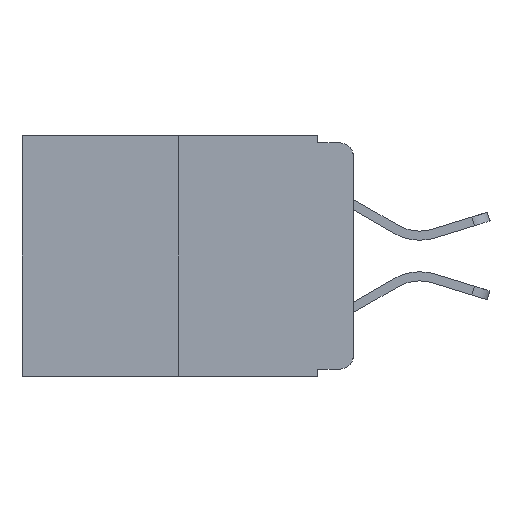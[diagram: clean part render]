
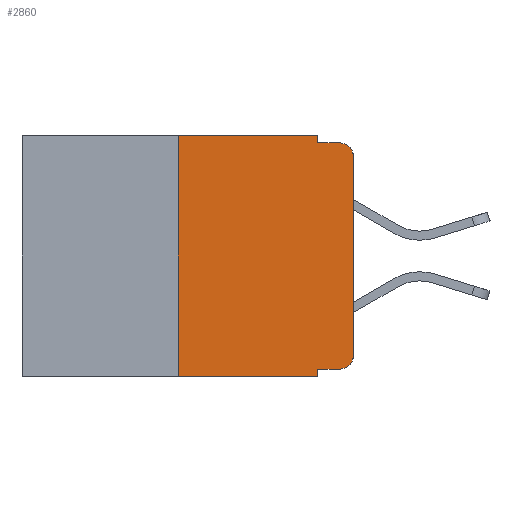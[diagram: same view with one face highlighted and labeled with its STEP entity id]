
A CAD part, left-side view. The second image highlights one B-rep face of the part: STEP entity #2860.
In plain terms, the highlighted planar face has unit normal (-1, 0, 0).
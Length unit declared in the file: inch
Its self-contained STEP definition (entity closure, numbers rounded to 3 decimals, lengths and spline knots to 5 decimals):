
#567 = EDGE_CURVE ( 'NONE', #4420, #1802, #23618, .T. ) ;
#629 = DIRECTION ( 'NONE',  ( 0., -1., 0. ) ) ;
#765 = VECTOR ( 'NONE', #10730, 39.37008 ) ;
#937 = DIRECTION ( 'NONE',  ( 0., -1., 0. ) ) ;
#1701 = DIRECTION ( 'NONE',  ( 0., 0., -1. ) ) ;
#1780 = PLANE ( 'NONE',  #20374 ) ;
#1802 = VERTEX_POINT ( 'NONE', #21354 ) ;
#2081 = VERTEX_POINT ( 'NONE', #8287 ) ;
#2464 = CARTESIAN_POINT ( 'NONE',  ( 0., 0.25, 0. ) ) ;
#2860 = ADVANCED_FACE ( 'NONE', ( #14733 ), #1780, .F. ) ;
#2958 = ORIENTED_EDGE ( 'NONE', *, *, #16913, .T. ) ;
#3296 = CARTESIAN_POINT ( 'NONE',  ( 0., 0.473, -0.343 ) ) ;
#3781 = LINE ( 'NONE', #13181, #8583 ) ;
#3833 = ORIENTED_EDGE ( 'NONE', *, *, #10765, .T. ) ;
#4156 = DIRECTION ( 'NONE',  ( 0., 0., -1. ) ) ;
#4213 = CARTESIAN_POINT ( 'NONE',  ( 0., 0.051, 0. ) ) ;
#4263 = ORIENTED_EDGE ( 'NONE', *, *, #8889, .F. ) ;
#4420 = VERTEX_POINT ( 'NONE', #11607 ) ;
#5229 = VERTEX_POINT ( 'NONE', #19844 ) ;
#6064 = VECTOR ( 'NONE', #1701, 39.37008 ) ;
#6263 = AXIS2_PLACEMENT_3D ( 'NONE', #19991, #8086, #21983 ) ;
#6359 = VERTEX_POINT ( 'NONE', #23585 ) ;
#6403 = VECTOR ( 'NONE', #629, 39.37008 ) ;
#7287 = CIRCLE ( 'NONE', #6263, 0.02 ) ;
#7420 = EDGE_CURVE ( 'NONE', #21089, #2081, #14067, .T. ) ;
#7659 = VERTEX_POINT ( 'NONE', #18163 ) ;
#7988 = DIRECTION ( 'NONE',  ( 0., 0., -1. ) ) ;
#8014 = EDGE_CURVE ( 'NONE', #7659, #9208, #14339, .T. ) ;
#8022 = ORIENTED_EDGE ( 'NONE', *, *, #20008, .F. ) ;
#8086 = DIRECTION ( 'NONE',  ( -1., 0., 0. ) ) ;
#8094 = VERTEX_POINT ( 'NONE', #23302 ) ;
#8287 = CARTESIAN_POINT ( 'NONE',  ( 0., 0.051, -0.343 ) ) ;
#8583 = VECTOR ( 'NONE', #937, 39.37008 ) ;
#8889 = EDGE_CURVE ( 'NONE', #1802, #13625, #21389, .T. ) ;
#9068 = VECTOR ( 'NONE', #4156, 39.37008 ) ;
#9083 = EDGE_CURVE ( 'NONE', #5229, #4420, #17061, .T. ) ;
#9143 = CARTESIAN_POINT ( 'NONE',  ( 0., 0., 0. ) ) ;
#9208 = VERTEX_POINT ( 'NONE', #17302 ) ;
#9276 = CARTESIAN_POINT ( 'NONE',  ( 0., 0.02, -0.313 ) ) ;
#10280 = ORIENTED_EDGE ( 'NONE', *, *, #9083, .F. ) ;
#10319 = CARTESIAN_POINT ( 'NONE',  ( 0., 0.051, -0.01 ) ) ;
#10730 = DIRECTION ( 'NONE',  ( 0., 0., 1. ) ) ;
#10765 = EDGE_CURVE ( 'NONE', #6359, #7659, #3781, .T. ) ;
#11051 = AXIS2_PLACEMENT_3D ( 'NONE', #9276, #23130, #11305 ) ;
#11305 = DIRECTION ( 'NONE',  ( 0., 0., -1. ) ) ;
#11607 = CARTESIAN_POINT ( 'NONE',  ( 0., 0.051, 0. ) ) ;
#11687 = LINE ( 'NONE', #2464, #765 ) ;
#11967 = CARTESIAN_POINT ( 'NONE',  ( 0., 0.473, 0. ) ) ;
#12489 = CARTESIAN_POINT ( 'NONE',  ( 0., 0.25, -0.343 ) ) ;
#12809 = VECTOR ( 'NONE', #21349, 39.37008 ) ;
#13025 = CARTESIAN_POINT ( 'NONE',  ( 0., 0.02, -0.01 ) ) ;
#13181 = CARTESIAN_POINT ( 'NONE',  ( 0., 0.051, -0.333 ) ) ;
#13625 = VERTEX_POINT ( 'NONE', #13025 ) ;
#13739 = LINE ( 'NONE', #9143, #17136 ) ;
#13892 = CARTESIAN_POINT ( 'NONE',  ( 0., 0.051, 0. ) ) ;
#14033 = EDGE_LOOP ( 'NONE', ( #23621, #2958, #4263, #16230, #10280, #8022, #25647, #21721, #3833, #21695 ) ) ;
#14067 = LINE ( 'NONE', #3296, #12809 ) ;
#14339 = CIRCLE ( 'NONE', #11051, 0.02 ) ;
#14733 = FACE_OUTER_BOUND ( 'NONE', #14033, .T. ) ;
#14758 = EDGE_CURVE ( 'NONE', #6359, #2081, #17373, .T. ) ;
#16230 = ORIENTED_EDGE ( 'NONE', *, *, #567, .F. ) ;
#16756 = VECTOR ( 'NONE', #22137, 39.37008 ) ;
#16913 = EDGE_CURVE ( 'NONE', #8094, #13625, #7287, .T. ) ;
#17061 = LINE ( 'NONE', #18678, #6403 ) ;
#17136 = VECTOR ( 'NONE', #24931, 39.37008 ) ;
#17302 = CARTESIAN_POINT ( 'NONE',  ( 0., 0., -0.313 ) ) ;
#17373 = LINE ( 'NONE', #13892, #6064 ) ;
#18163 = CARTESIAN_POINT ( 'NONE',  ( 0., 0.02, -0.333 ) ) ;
#18678 = CARTESIAN_POINT ( 'NONE',  ( 0., 0.473, 0. ) ) ;
#19844 = CARTESIAN_POINT ( 'NONE',  ( 0., 0.25, 0. ) ) ;
#19919 = DIRECTION ( 'NONE',  ( 1., 0., 0. ) ) ;
#19991 = CARTESIAN_POINT ( 'NONE',  ( 0., 0.02, -0.03 ) ) ;
#20008 = EDGE_CURVE ( 'NONE', #21089, #5229, #11687, .T. ) ;
#20374 = AXIS2_PLACEMENT_3D ( 'NONE', #11967, #19919, #7988 ) ;
#21089 = VERTEX_POINT ( 'NONE', #12489 ) ;
#21349 = DIRECTION ( 'NONE',  ( 0., -1., 0. ) ) ;
#21354 = CARTESIAN_POINT ( 'NONE',  ( 0., 0.051, -0.01 ) ) ;
#21389 = LINE ( 'NONE', #10319, #16756 ) ;
#21695 = ORIENTED_EDGE ( 'NONE', *, *, #8014, .T. ) ;
#21721 = ORIENTED_EDGE ( 'NONE', *, *, #14758, .F. ) ;
#21983 = DIRECTION ( 'NONE',  ( 0., 0., -1. ) ) ;
#22137 = DIRECTION ( 'NONE',  ( 0., -1., 0. ) ) ;
#23130 = DIRECTION ( 'NONE',  ( -1., 0., 0. ) ) ;
#23302 = CARTESIAN_POINT ( 'NONE',  ( 0., 0., -0.03 ) ) ;
#23585 = CARTESIAN_POINT ( 'NONE',  ( 0., 0.051, -0.333 ) ) ;
#23618 = LINE ( 'NONE', #4213, #9068 ) ;
#23621 = ORIENTED_EDGE ( 'NONE', *, *, #24782, .T. ) ;
#24782 = EDGE_CURVE ( 'NONE', #9208, #8094, #13739, .T. ) ;
#24931 = DIRECTION ( 'NONE',  ( 0., 0., 1. ) ) ;
#25647 = ORIENTED_EDGE ( 'NONE', *, *, #7420, .T. ) ;
